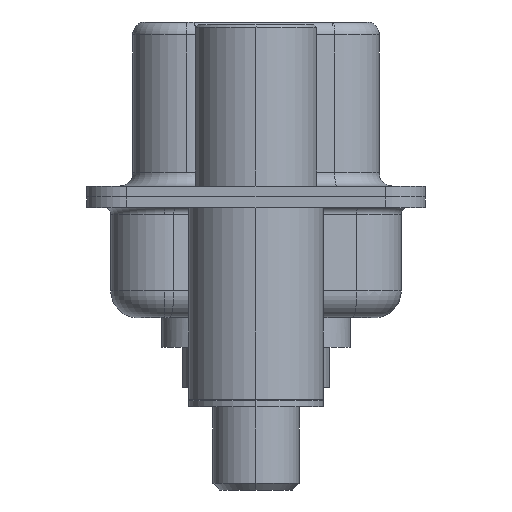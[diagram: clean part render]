
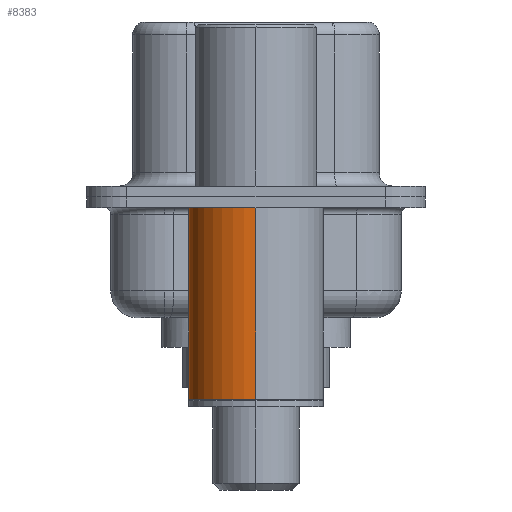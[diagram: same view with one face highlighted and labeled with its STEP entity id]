
A CAD part, left-side view. The second image highlights one B-rep face of the part: STEP entity #8383.
In plain terms, the highlighted cylindrical face has radius 2.5 mm (diameter 5 mm), a partial arc.
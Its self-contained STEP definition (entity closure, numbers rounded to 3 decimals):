
#432 = CARTESIAN_POINT ( 'NONE',  ( -2.5, 0., -0.4 ) ) ;
#680 = VERTEX_POINT ( 'NONE', #432 ) ;
#923 = CARTESIAN_POINT ( 'NONE',  ( 2.5, 0., -0.4 ) ) ;
#1476 = CARTESIAN_POINT ( 'NONE',  ( -2.5, 0., 0.581 ) ) ;
#2452 = CARTESIAN_POINT ( 'NONE',  ( 0., 0., -7.525 ) ) ;
#2710 = CARTESIAN_POINT ( 'NONE',  ( 0., 0., -0.4 ) ) ;
#2875 = DIRECTION ( 'NONE',  ( 0., 0., 1. ) ) ;
#2971 = AXIS2_PLACEMENT_3D ( 'NONE', #18757, #2875, #22477 ) ;
#3212 = LINE ( 'NONE', #12012, #9590 ) ;
#3888 = CARTESIAN_POINT ( 'NONE',  ( 2.5, 0., -7.525 ) ) ;
#4262 = VERTEX_POINT ( 'NONE', #923 ) ;
#5487 = EDGE_CURVE ( 'NONE', #7170, #680, #18828, .T. ) ;
#7170 = VERTEX_POINT ( 'NONE', #13329 ) ;
#7564 = DIRECTION ( 'NONE',  ( 0., 0., 1. ) ) ;
#8101 = VERTEX_POINT ( 'NONE', #3888 ) ;
#8189 = CYLINDRICAL_SURFACE ( 'NONE', #2971, 2.5 ) ;
#8383 = ADVANCED_FACE ( 'NONE', ( #12399 ), #8189, .T. ) ;
#8728 = AXIS2_PLACEMENT_3D ( 'NONE', #2710, #11401, #13265 ) ;
#9590 = VECTOR ( 'NONE', #20920, 1000. ) ;
#9896 = VECTOR ( 'NONE', #10410, 1000. ) ;
#10410 = DIRECTION ( 'NONE',  ( 0., 0., 1. ) ) ;
#11323 = EDGE_LOOP ( 'NONE', ( #21257, #14521, #13271, #12465 ) ) ;
#11401 = DIRECTION ( 'NONE',  ( 0., 0., 1. ) ) ;
#11846 = AXIS2_PLACEMENT_3D ( 'NONE', #2452, #7564, #18324 ) ;
#12012 = CARTESIAN_POINT ( 'NONE',  ( 2.5, 0., 0.581 ) ) ;
#12399 = FACE_OUTER_BOUND ( 'NONE', #11323, .T. ) ;
#12465 = ORIENTED_EDGE ( 'NONE', *, *, #22997, .F. ) ;
#13265 = DIRECTION ( 'NONE',  ( 1., 0., 0. ) ) ;
#13271 = ORIENTED_EDGE ( 'NONE', *, *, #22197, .F. ) ;
#13329 = CARTESIAN_POINT ( 'NONE',  ( -2.5, 0., -7.525 ) ) ;
#14521 = ORIENTED_EDGE ( 'NONE', *, *, #5487, .T. ) ;
#17474 = CIRCLE ( 'NONE', #8728, 2.5 ) ;
#18324 = DIRECTION ( 'NONE',  ( 1., 0., 0. ) ) ;
#18757 = CARTESIAN_POINT ( 'NONE',  ( 0., 0., 0.581 ) ) ;
#18828 = LINE ( 'NONE', #1476, #9896 ) ;
#18893 = CIRCLE ( 'NONE', #11846, 2.5 ) ;
#20912 = EDGE_CURVE ( 'NONE', #8101, #7170, #18893, .T. ) ;
#20920 = DIRECTION ( 'NONE',  ( 0., 0., 1. ) ) ;
#21257 = ORIENTED_EDGE ( 'NONE', *, *, #20912, .T. ) ;
#22197 = EDGE_CURVE ( 'NONE', #4262, #680, #17474, .T. ) ;
#22477 = DIRECTION ( 'NONE',  ( 1., 0., 0. ) ) ;
#22997 = EDGE_CURVE ( 'NONE', #8101, #4262, #3212, .T. ) ;
